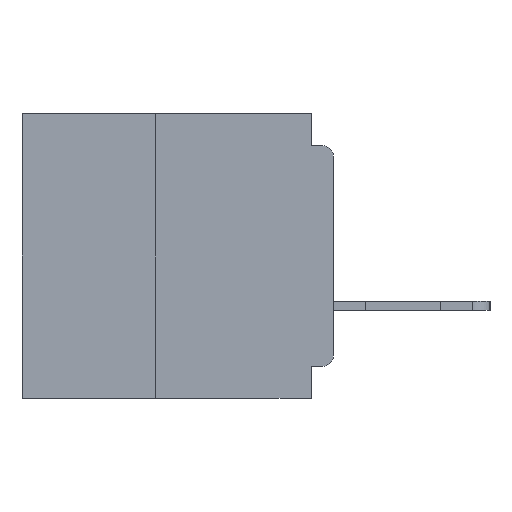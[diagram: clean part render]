
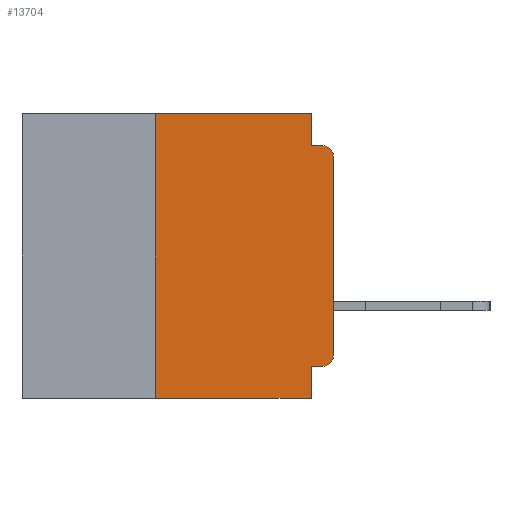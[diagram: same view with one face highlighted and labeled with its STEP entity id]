
A CAD part, left-side view. The second image highlights one B-rep face of the part: STEP entity #13704.
In plain terms, the highlighted planar face has unit normal (-1, 0, 0).
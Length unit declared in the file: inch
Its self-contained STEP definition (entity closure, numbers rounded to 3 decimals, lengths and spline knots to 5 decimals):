
#363 = DIRECTION ( 'NONE',  ( 0., -1., 0. ) ) ;
#366 = VERTEX_POINT ( 'NONE', #5657 ) ;
#390 = ORIENTED_EDGE ( 'NONE', *, *, #33515, .T. ) ;
#766 = VERTEX_POINT ( 'NONE', #28887 ) ;
#1506 = CARTESIAN_POINT ( 'NONE',  ( 0., 0., -0.045 ) ) ;
#1513 = AXIS2_PLACEMENT_3D ( 'NONE', #28665, #9446, #31782 ) ;
#1751 = CARTESIAN_POINT ( 'NONE',  ( 0., 0.015, -0.355 ) ) ;
#1866 = LINE ( 'NONE', #6299, #18051 ) ;
#2143 = ORIENTED_EDGE ( 'NONE', *, *, #2628, .T. ) ;
#2403 = DIRECTION ( 'NONE',  ( 0., 0., -1. ) ) ;
#2597 = CARTESIAN_POINT ( 'NONE',  ( 0., 0.437, 0. ) ) ;
#2628 = EDGE_CURVE ( 'NONE', #28413, #366, #17808, .T. ) ;
#3466 = ORIENTED_EDGE ( 'NONE', *, *, #38979, .F. ) ;
#4880 = ORIENTED_EDGE ( 'NONE', *, *, #29113, .F. ) ;
#4985 = CARTESIAN_POINT ( 'NONE',  ( 0., 0.25, -0.4 ) ) ;
#4994 = VECTOR ( 'NONE', #40528, 39.37008 ) ;
#5052 = VERTEX_POINT ( 'NONE', #4985 ) ;
#5657 = CARTESIAN_POINT ( 'NONE',  ( 0., 0., -0.34 ) ) ;
#5690 = EDGE_CURVE ( 'NONE', #766, #25268, #18115, .T. ) ;
#6003 = CARTESIAN_POINT ( 'NONE',  ( 0., 0.25, -0.4 ) ) ;
#6299 = CARTESIAN_POINT ( 'NONE',  ( 0., 0., 0. ) ) ;
#6649 = ORIENTED_EDGE ( 'NONE', *, *, #5690, .F. ) ;
#7824 = LINE ( 'NONE', #16467, #24992 ) ;
#8331 = VECTOR ( 'NONE', #36620, 39.37008 ) ;
#8495 = AXIS2_PLACEMENT_3D ( 'NONE', #38100, #19270, #41230 ) ;
#9296 = ORIENTED_EDGE ( 'NONE', *, *, #24091, .F. ) ;
#9446 = DIRECTION ( 'NONE',  ( -1., 0., 0. ) ) ;
#9539 = DIRECTION ( 'NONE',  ( 0., 0., 1. ) ) ;
#9904 = ORIENTED_EDGE ( 'NONE', *, *, #33715, .F. ) ;
#11731 = LINE ( 'NONE', #18520, #19321 ) ;
#11892 = CARTESIAN_POINT ( 'NONE',  ( 0., 0.031, -0.045 ) ) ;
#12832 = CARTESIAN_POINT ( 'NONE',  ( 0., 0.031, -0.4 ) ) ;
#13704 = ADVANCED_FACE ( 'NONE', ( #23029 ), #34571, .F. ) ;
#15584 = DIRECTION ( 'NONE',  ( 1., 0., 0. ) ) ;
#16132 = CIRCLE ( 'NONE', #1513, 0.015 ) ;
#16467 = CARTESIAN_POINT ( 'NONE',  ( 0., 0.437, -0.4 ) ) ;
#16716 = EDGE_CURVE ( 'NONE', #21731, #41139, #16132, .T. ) ;
#17808 = CIRCLE ( 'NONE', #8495, 0.015 ) ;
#18051 = VECTOR ( 'NONE', #9539, 39.37008 ) ;
#18115 = LINE ( 'NONE', #37357, #41215 ) ;
#18520 = CARTESIAN_POINT ( 'NONE',  ( 0., 0.031, 0. ) ) ;
#18546 = CARTESIAN_POINT ( 'NONE',  ( 0., 0.437, 0. ) ) ;
#19056 = AXIS2_PLACEMENT_3D ( 'NONE', #2597, #15584, #37692 ) ;
#19202 = VERTEX_POINT ( 'NONE', #20659 ) ;
#19270 = DIRECTION ( 'NONE',  ( -1., 0., 0. ) ) ;
#19321 = VECTOR ( 'NONE', #2403, 39.37008 ) ;
#20520 = EDGE_LOOP ( 'NONE', ( #31609, #38474, #36815, #4880, #9296, #3466, #390, #6649, #9904, #2143 ) ) ;
#20659 = CARTESIAN_POINT ( 'NONE',  ( 0., 0.25, 0. ) ) ;
#21731 = VERTEX_POINT ( 'NONE', #36396 ) ;
#22245 = VERTEX_POINT ( 'NONE', #11892 ) ;
#23029 = FACE_OUTER_BOUND ( 'NONE', #20520, .T. ) ;
#23659 = LINE ( 'NONE', #1506, #30006 ) ;
#24091 = EDGE_CURVE ( 'NONE', #19202, #24977, #30551, .T. ) ;
#24977 = VERTEX_POINT ( 'NONE', #36700 ) ;
#24992 = VECTOR ( 'NONE', #363, 39.37008 ) ;
#25268 = VERTEX_POINT ( 'NONE', #12832 ) ;
#25464 = LINE ( 'NONE', #39739, #8331 ) ;
#25542 = LINE ( 'NONE', #6003, #41096 ) ;
#25551 = EDGE_CURVE ( 'NONE', #22245, #41139, #23659, .T. ) ;
#25851 = EDGE_CURVE ( 'NONE', #366, #21731, #1866, .T. ) ;
#28413 = VERTEX_POINT ( 'NONE', #1751 ) ;
#28665 = CARTESIAN_POINT ( 'NONE',  ( 0., 0.015, -0.06 ) ) ;
#28887 = CARTESIAN_POINT ( 'NONE',  ( 0., 0.031, -0.355 ) ) ;
#29113 = EDGE_CURVE ( 'NONE', #24977, #22245, #11731, .T. ) ;
#30006 = VECTOR ( 'NONE', #36651, 39.37008 ) ;
#30551 = LINE ( 'NONE', #18546, #4994 ) ;
#31602 = DIRECTION ( 'NONE',  ( 0., 0., 1. ) ) ;
#31609 = ORIENTED_EDGE ( 'NONE', *, *, #25851, .T. ) ;
#31782 = DIRECTION ( 'NONE',  ( 0., 0., -1. ) ) ;
#33515 = EDGE_CURVE ( 'NONE', #5052, #25268, #7824, .T. ) ;
#33715 = EDGE_CURVE ( 'NONE', #28413, #766, #25464, .T. ) ;
#34571 = PLANE ( 'NONE',  #19056 ) ;
#36396 = CARTESIAN_POINT ( 'NONE',  ( 0., 0., -0.06 ) ) ;
#36620 = DIRECTION ( 'NONE',  ( 0., 1., 0. ) ) ;
#36651 = DIRECTION ( 'NONE',  ( 0., -1., 0. ) ) ;
#36700 = CARTESIAN_POINT ( 'NONE',  ( 0., 0.031, 0. ) ) ;
#36815 = ORIENTED_EDGE ( 'NONE', *, *, #25551, .F. ) ;
#37357 = CARTESIAN_POINT ( 'NONE',  ( 0., 0.031, -0.4 ) ) ;
#37491 = DIRECTION ( 'NONE',  ( 0., 0., -1. ) ) ;
#37692 = DIRECTION ( 'NONE',  ( 0., 0., -1. ) ) ;
#38100 = CARTESIAN_POINT ( 'NONE',  ( 0., 0.015, -0.34 ) ) ;
#38474 = ORIENTED_EDGE ( 'NONE', *, *, #16716, .T. ) ;
#38979 = EDGE_CURVE ( 'NONE', #5052, #19202, #25542, .T. ) ;
#39739 = CARTESIAN_POINT ( 'NONE',  ( 0., 0., -0.355 ) ) ;
#39859 = CARTESIAN_POINT ( 'NONE',  ( 0., 0.015, -0.045 ) ) ;
#40528 = DIRECTION ( 'NONE',  ( 0., -1., 0. ) ) ;
#41096 = VECTOR ( 'NONE', #31602, 39.37008 ) ;
#41139 = VERTEX_POINT ( 'NONE', #39859 ) ;
#41215 = VECTOR ( 'NONE', #37491, 39.37008 ) ;
#41230 = DIRECTION ( 'NONE',  ( 0., 0., -1. ) ) ;
